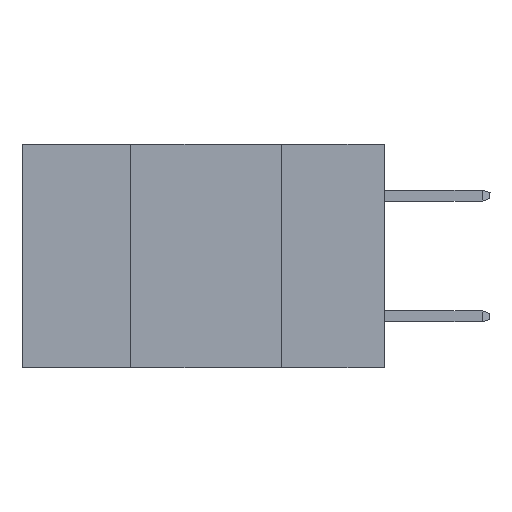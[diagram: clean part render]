
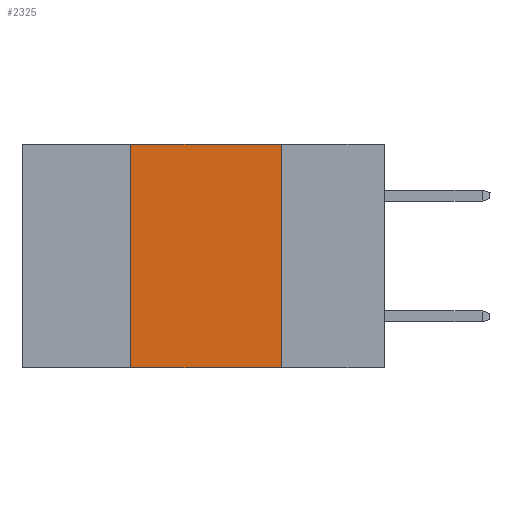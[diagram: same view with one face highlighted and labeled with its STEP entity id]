
A CAD part, left-side view. The second image highlights one B-rep face of the part: STEP entity #2325.
In plain terms, the highlighted planar face has unit normal (-1, 0, 0).
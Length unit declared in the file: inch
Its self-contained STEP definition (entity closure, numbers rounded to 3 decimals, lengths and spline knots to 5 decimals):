
#15 = ORIENTED_EDGE ( 'NONE', *, *, #20873, .T. ) ;
#1899 = PLANE ( 'NONE',  #4212 ) ;
#2215 = ORIENTED_EDGE ( 'NONE', *, *, #21532, .F. ) ;
#2325 = ADVANCED_FACE ( 'NONE', ( #7551 ), #1899, .F. ) ;
#2503 = DIRECTION ( 'NONE',  ( 0., -1., 0. ) ) ;
#2685 = LINE ( 'NONE', #22240, #27992 ) ;
#2717 = VERTEX_POINT ( 'NONE', #28781 ) ;
#3316 = CARTESIAN_POINT ( 'NONE',  ( 0., 0.42, 0. ) ) ;
#4212 = AXIS2_PLACEMENT_3D ( 'NONE', #25717, #20389, #15590 ) ;
#5177 = EDGE_CURVE ( 'NONE', #16719, #2717, #14771, .T. ) ;
#7551 = FACE_OUTER_BOUND ( 'NONE', #22387, .T. ) ;
#10732 = CARTESIAN_POINT ( 'NONE',  ( 0., 0.17, -0.37 ) ) ;
#10793 = CARTESIAN_POINT ( 'NONE',  ( 0., 0.42, -0.37 ) ) ;
#11349 = LINE ( 'NONE', #30594, #24339 ) ;
#12328 = VECTOR ( 'NONE', #2503, 39.37008 ) ;
#12785 = CARTESIAN_POINT ( 'NONE',  ( 0., 0.17, 0. ) ) ;
#14771 = LINE ( 'NONE', #3316, #16303 ) ;
#15590 = DIRECTION ( 'NONE',  ( 0., 0., -1. ) ) ;
#16303 = VECTOR ( 'NONE', #24420, 39.37008 ) ;
#16510 = DIRECTION ( 'NONE',  ( 0., 0., -1. ) ) ;
#16719 = VERTEX_POINT ( 'NONE', #10793 ) ;
#17138 = LINE ( 'NONE', #24120, #12328 ) ;
#18239 = EDGE_CURVE ( 'NONE', #19687, #20966, #11349, .T. ) ;
#18616 = ORIENTED_EDGE ( 'NONE', *, *, #18239, .F. ) ;
#19687 = VERTEX_POINT ( 'NONE', #12785 ) ;
#20389 = DIRECTION ( 'NONE',  ( 1., 0., 0. ) ) ;
#20873 = EDGE_CURVE ( 'NONE', #16719, #20966, #2685, .T. ) ;
#20966 = VERTEX_POINT ( 'NONE', #10732 ) ;
#21532 = EDGE_CURVE ( 'NONE', #2717, #19687, #17138, .T. ) ;
#22240 = CARTESIAN_POINT ( 'NONE',  ( 0., 0.6, -0.37 ) ) ;
#22387 = EDGE_LOOP ( 'NONE', ( #18616, #2215, #26637, #15 ) ) ;
#24120 = CARTESIAN_POINT ( 'NONE',  ( 0., 0.6, 0. ) ) ;
#24339 = VECTOR ( 'NONE', #16510, 39.37008 ) ;
#24420 = DIRECTION ( 'NONE',  ( 0., 0., 1. ) ) ;
#24641 = DIRECTION ( 'NONE',  ( 0., -1., 0. ) ) ;
#25717 = CARTESIAN_POINT ( 'NONE',  ( 0., 0.6, 0. ) ) ;
#26637 = ORIENTED_EDGE ( 'NONE', *, *, #5177, .F. ) ;
#27992 = VECTOR ( 'NONE', #24641, 39.37008 ) ;
#28781 = CARTESIAN_POINT ( 'NONE',  ( 0., 0.42, 0. ) ) ;
#30594 = CARTESIAN_POINT ( 'NONE',  ( 0., 0.17, 0. ) ) ;
